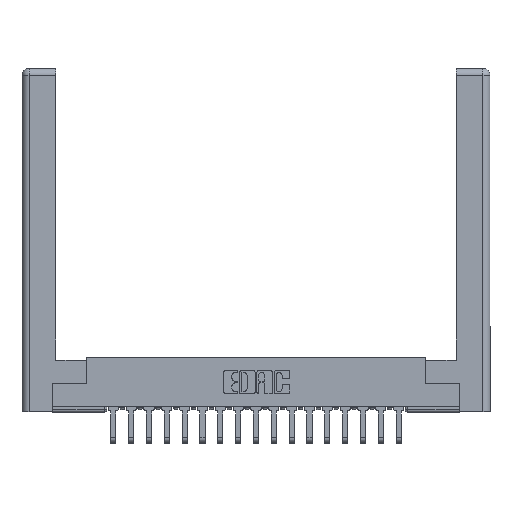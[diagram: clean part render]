
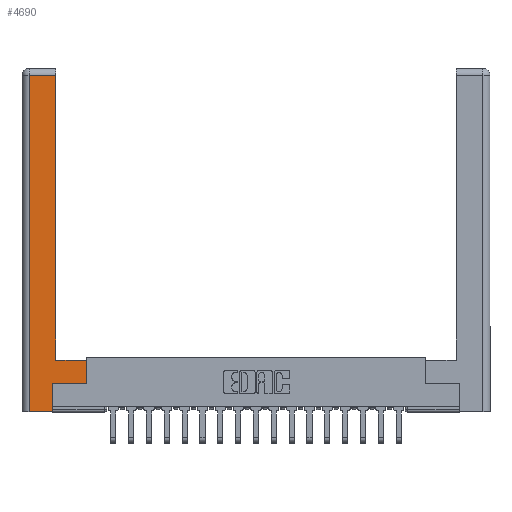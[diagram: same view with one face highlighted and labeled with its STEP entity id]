
A CAD part, top view. The second image highlights one B-rep face of the part: STEP entity #4690.
In plain terms, the highlighted planar face has unit normal (0, 0, 1).
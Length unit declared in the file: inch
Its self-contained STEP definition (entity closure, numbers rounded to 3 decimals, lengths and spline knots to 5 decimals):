
#210 = VECTOR ( 'NONE', #15500, 39.37008 ) ;
#412 = CARTESIAN_POINT ( 'NONE',  ( 0.265, 0.245, 0. ) ) ;
#669 = ORIENTED_EDGE ( 'NONE', *, *, #7293, .T. ) ;
#837 = CARTESIAN_POINT ( 'NONE',  ( 0.565, 0.45, 0. ) ) ;
#968 = DIRECTION ( 'NONE',  ( 0., 0., -1. ) ) ;
#1168 = CARTESIAN_POINT ( 'NONE',  ( 0.265, 0., 0. ) ) ;
#1206 = AXIS2_PLACEMENT_3D ( 'NONE', #10375, #968, #19735 ) ;
#1253 = LINE ( 'NONE', #10115, #7640 ) ;
#1537 = VECTOR ( 'NONE', #19322, 39.37008 ) ;
#1699 = VECTOR ( 'NONE', #14858, 39.37008 ) ;
#1758 = CARTESIAN_POINT ( 'NONE',  ( 0.0615, 2.94, 0. ) ) ;
#1884 = EDGE_CURVE ( 'NONE', #3719, #7401, #4376, .T. ) ;
#2341 = DIRECTION ( 'NONE',  ( 0., 1., 0. ) ) ;
#2448 = VERTEX_POINT ( 'NONE', #6334 ) ;
#2891 = VERTEX_POINT ( 'NONE', #1168 ) ;
#2963 = CARTESIAN_POINT ( 'NONE',  ( 0.0615, 0., 0. ) ) ;
#3710 = ORIENTED_EDGE ( 'NONE', *, *, #18803, .T. ) ;
#3719 = VERTEX_POINT ( 'NONE', #1758 ) ;
#3818 = ORIENTED_EDGE ( 'NONE', *, *, #9204, .T. ) ;
#3861 = CARTESIAN_POINT ( 'NONE',  ( 0.265, 0.245, 0. ) ) ;
#4216 = CARTESIAN_POINT ( 'NONE',  ( 0.565, 0.245, 0. ) ) ;
#4376 = LINE ( 'NONE', #17786, #1699 ) ;
#4490 = CARTESIAN_POINT ( 'NONE',  ( 0.295, 2.94, 0. ) ) ;
#4690 = ADVANCED_FACE ( 'NONE', ( #15097 ), #11743, .F. ) ;
#5182 = DIRECTION ( 'NONE',  ( -1., 0., 0. ) ) ;
#5577 = LINE ( 'NONE', #11793, #17850 ) ;
#5619 = LINE ( 'NONE', #20156, #15444 ) ;
#5729 = LINE ( 'NONE', #412, #1537 ) ;
#6156 = VECTOR ( 'NONE', #14997, 39.37008 ) ;
#6172 = ORIENTED_EDGE ( 'NONE', *, *, #9886, .T. ) ;
#6334 = CARTESIAN_POINT ( 'NONE',  ( 0.565, 0.45, 0. ) ) ;
#6723 = VERTEX_POINT ( 'NONE', #12364 ) ;
#7293 = EDGE_CURVE ( 'NONE', #17043, #6723, #16687, .T. ) ;
#7401 = VERTEX_POINT ( 'NONE', #2963 ) ;
#7640 = VECTOR ( 'NONE', #2341, 39.37008 ) ;
#7715 = ORIENTED_EDGE ( 'NONE', *, *, #1884, .T. ) ;
#8342 = CARTESIAN_POINT ( 'NONE',  ( 0.0615, 2.94, 0. ) ) ;
#8523 = VERTEX_POINT ( 'NONE', #14021 ) ;
#8705 = DIRECTION ( 'NONE',  ( 1., 0., 0. ) ) ;
#9115 = ORIENTED_EDGE ( 'NONE', *, *, #16050, .T. ) ;
#9204 = EDGE_CURVE ( 'NONE', #15067, #3719, #16787, .T. ) ;
#9858 = EDGE_CURVE ( 'NONE', #8523, #15067, #1253, .T. ) ;
#9886 = EDGE_CURVE ( 'NONE', #6723, #2448, #10365, .T. ) ;
#10115 = CARTESIAN_POINT ( 'NONE',  ( 0.295, 3., 0. ) ) ;
#10365 = LINE ( 'NONE', #837, #6156 ) ;
#10375 = CARTESIAN_POINT ( 'NONE',  ( 0., 0., 0. ) ) ;
#11743 = PLANE ( 'NONE',  #1206 ) ;
#11793 = CARTESIAN_POINT ( 'NONE',  ( 0.265, 0., 0. ) ) ;
#12364 = CARTESIAN_POINT ( 'NONE',  ( 0.565, 0.245, 0. ) ) ;
#14021 = CARTESIAN_POINT ( 'NONE',  ( 0.295, 0.45, 0. ) ) ;
#14858 = DIRECTION ( 'NONE',  ( 0., -1., 0. ) ) ;
#14997 = DIRECTION ( 'NONE',  ( 0., 1., 0. ) ) ;
#15067 = VERTEX_POINT ( 'NONE', #4490 ) ;
#15097 = FACE_OUTER_BOUND ( 'NONE', #16353, .T. ) ;
#15286 = DIRECTION ( 'NONE',  ( -1., 0., 0. ) ) ;
#15444 = VECTOR ( 'NONE', #15286, 39.37008 ) ;
#15500 = DIRECTION ( 'NONE',  ( 1., 0., 0. ) ) ;
#15793 = VECTOR ( 'NONE', #5182, 39.37008 ) ;
#16050 = EDGE_CURVE ( 'NONE', #2448, #8523, #5619, .T. ) ;
#16353 = EDGE_LOOP ( 'NONE', ( #20268, #3818, #7715, #17812, #3710, #669, #6172, #9115 ) ) ;
#16687 = LINE ( 'NONE', #4216, #210 ) ;
#16787 = LINE ( 'NONE', #8342, #15793 ) ;
#17043 = VERTEX_POINT ( 'NONE', #3861 ) ;
#17073 = EDGE_CURVE ( 'NONE', #7401, #2891, #5577, .T. ) ;
#17786 = CARTESIAN_POINT ( 'NONE',  ( 0.0615, 0., 0. ) ) ;
#17812 = ORIENTED_EDGE ( 'NONE', *, *, #17073, .T. ) ;
#17850 = VECTOR ( 'NONE', #8705, 39.37008 ) ;
#18803 = EDGE_CURVE ( 'NONE', #2891, #17043, #5729, .T. ) ;
#19322 = DIRECTION ( 'NONE',  ( 0., 1., 0. ) ) ;
#19735 = DIRECTION ( 'NONE',  ( -1., 0., 0. ) ) ;
#20156 = CARTESIAN_POINT ( 'NONE',  ( 0.295, 0.45, 0. ) ) ;
#20268 = ORIENTED_EDGE ( 'NONE', *, *, #9858, .T. ) ;
